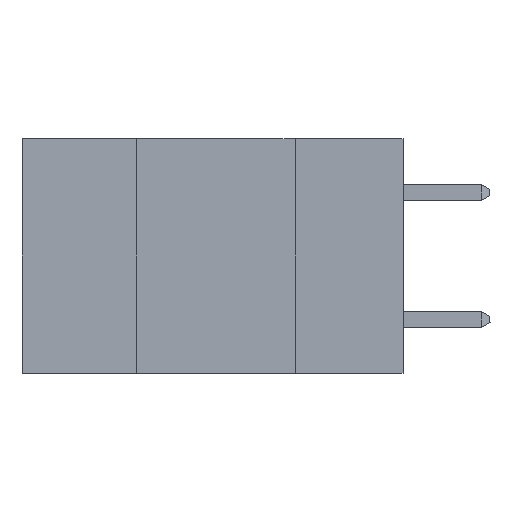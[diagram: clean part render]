
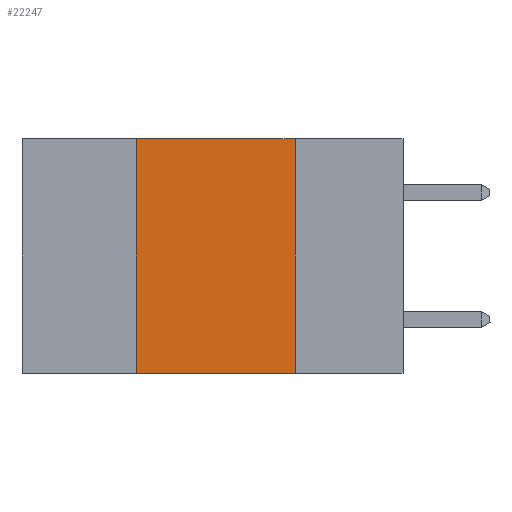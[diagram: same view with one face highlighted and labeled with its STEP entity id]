
A CAD part, left-side view. The second image highlights one B-rep face of the part: STEP entity #22247.
In plain terms, the highlighted planar face has unit normal (-1, 0, 0).
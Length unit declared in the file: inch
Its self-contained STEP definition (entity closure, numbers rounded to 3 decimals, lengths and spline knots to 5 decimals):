
#379 = CARTESIAN_POINT ( 'NONE',  ( 0., 0.42, 0. ) ) ;
#404 = ORIENTED_EDGE ( 'NONE', *, *, #5154, .F. ) ;
#901 = LINE ( 'NONE', #379, #1778 ) ;
#1778 = VECTOR ( 'NONE', #2272, 39.37008 ) ;
#2018 = VERTEX_POINT ( 'NONE', #5231 ) ;
#2272 = DIRECTION ( 'NONE',  ( 0., 0., 1. ) ) ;
#2459 = LINE ( 'NONE', #17562, #21628 ) ;
#3265 = VERTEX_POINT ( 'NONE', #6232 ) ;
#5154 = EDGE_CURVE ( 'NONE', #15965, #20190, #10356, .T. ) ;
#5231 = CARTESIAN_POINT ( 'NONE',  ( 0., 0.17, -0.37 ) ) ;
#6232 = CARTESIAN_POINT ( 'NONE',  ( 0., 0.42, -0.37 ) ) ;
#6635 = DIRECTION ( 'NONE',  ( 0., -1., 0. ) ) ;
#8324 = CARTESIAN_POINT ( 'NONE',  ( 0., 0.6, 0. ) ) ;
#8445 = FACE_OUTER_BOUND ( 'NONE', #12320, .T. ) ;
#9251 = DIRECTION ( 'NONE',  ( 0., 0., -1. ) ) ;
#9892 = LINE ( 'NONE', #14740, #20878 ) ;
#10356 = LINE ( 'NONE', #8324, #18742 ) ;
#10434 = CARTESIAN_POINT ( 'NONE',  ( 0., 0.17, 0. ) ) ;
#11994 = ORIENTED_EDGE ( 'NONE', *, *, #18822, .T. ) ;
#12320 = EDGE_LOOP ( 'NONE', ( #14685, #404, #18767, #11994 ) ) ;
#13206 = CARTESIAN_POINT ( 'NONE',  ( 0., 0.6, 0. ) ) ;
#14578 = DIRECTION ( 'NONE',  ( 0., 0., -1. ) ) ;
#14685 = ORIENTED_EDGE ( 'NONE', *, *, #24000, .F. ) ;
#14740 = CARTESIAN_POINT ( 'NONE',  ( 0., 0.17, 0. ) ) ;
#15163 = EDGE_CURVE ( 'NONE', #3265, #15965, #901, .T. ) ;
#15965 = VERTEX_POINT ( 'NONE', #21467 ) ;
#16854 = DIRECTION ( 'NONE',  ( 1., 0., 0. ) ) ;
#17562 = CARTESIAN_POINT ( 'NONE',  ( 0., 0.6, -0.37 ) ) ;
#18742 = VECTOR ( 'NONE', #6635, 39.37008 ) ;
#18767 = ORIENTED_EDGE ( 'NONE', *, *, #15163, .F. ) ;
#18822 = EDGE_CURVE ( 'NONE', #3265, #2018, #2459, .T. ) ;
#19544 = AXIS2_PLACEMENT_3D ( 'NONE', #13206, #16854, #9251 ) ;
#20190 = VERTEX_POINT ( 'NONE', #10434 ) ;
#20581 = PLANE ( 'NONE',  #19544 ) ;
#20878 = VECTOR ( 'NONE', #14578, 39.37008 ) ;
#21300 = DIRECTION ( 'NONE',  ( 0., -1., 0. ) ) ;
#21467 = CARTESIAN_POINT ( 'NONE',  ( 0., 0.42, 0. ) ) ;
#21628 = VECTOR ( 'NONE', #21300, 39.37008 ) ;
#22247 = ADVANCED_FACE ( 'NONE', ( #8445 ), #20581, .F. ) ;
#24000 = EDGE_CURVE ( 'NONE', #20190, #2018, #9892, .T. ) ;
